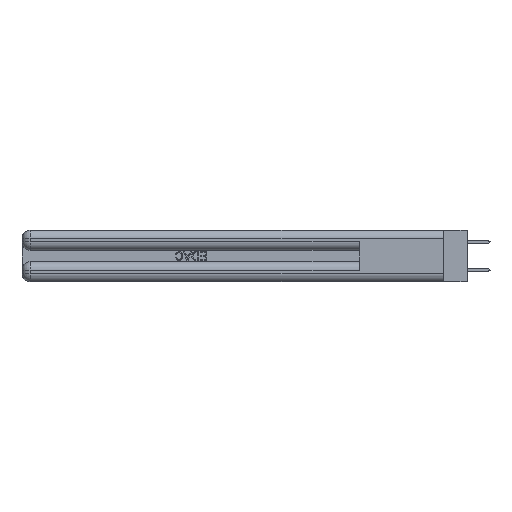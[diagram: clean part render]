
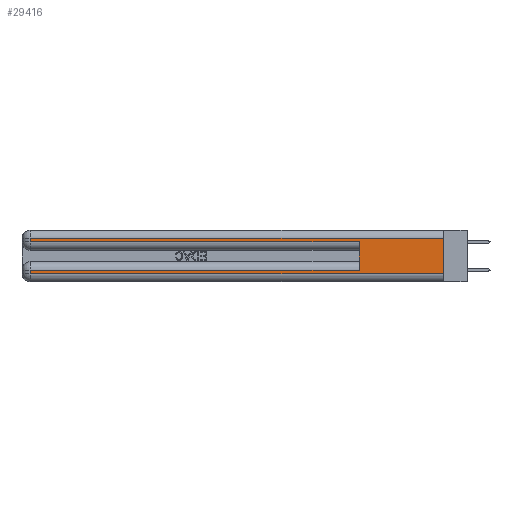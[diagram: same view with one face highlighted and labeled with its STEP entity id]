
A CAD part, left-side view. The second image highlights one B-rep face of the part: STEP entity #29416.
In plain terms, the highlighted planar face has unit normal (-1, 0, 0).
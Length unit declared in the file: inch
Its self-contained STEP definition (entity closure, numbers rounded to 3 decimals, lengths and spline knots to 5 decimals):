
#1865 = EDGE_CURVE ( 'NONE', #43558, #9555, #14047, .T. ) ;
#2271 = AXIS2_PLACEMENT_3D ( 'NONE', #34274, #13079, #16820 ) ;
#2490 = VERTEX_POINT ( 'NONE', #23198 ) ;
#3657 = DIRECTION ( 'NONE',  ( 0., -1., 0. ) ) ;
#5182 = VECTOR ( 'NONE', #38773, 39.37008 ) ;
#5580 = CARTESIAN_POINT ( 'NONE',  ( 0., 0., 0.31 ) ) ;
#7003 = LINE ( 'NONE', #28670, #10877 ) ;
#7326 = ORIENTED_EDGE ( 'NONE', *, *, #19585, .T. ) ;
#7489 = LINE ( 'NONE', #20297, #21971 ) ;
#7851 = DIRECTION ( 'NONE',  ( 0., 0., -1. ) ) ;
#9555 = VERTEX_POINT ( 'NONE', #19583 ) ;
#9772 = VECTOR ( 'NONE', #13461, 39.37008 ) ;
#10008 = CARTESIAN_POINT ( 'NONE',  ( 0., 0.6, 0.085 ) ) ;
#10312 = EDGE_CURVE ( 'NONE', #43558, #22342, #7489, .T. ) ;
#10806 = LINE ( 'NONE', #34805, #19724 ) ;
#10877 = VECTOR ( 'NONE', #35688, 39.37008 ) ;
#13079 = DIRECTION ( 'NONE',  ( 1., 0., 0. ) ) ;
#13461 = DIRECTION ( 'NONE',  ( 0., 0., -1. ) ) ;
#14047 = LINE ( 'NONE', #35183, #5182 ) ;
#14263 = VERTEX_POINT ( 'NONE', #40095 ) ;
#14584 = VERTEX_POINT ( 'NONE', #35047 ) ;
#15767 = CARTESIAN_POINT ( 'NONE',  ( 0., 0., 0.285 ) ) ;
#16317 = EDGE_CURVE ( 'NONE', #22370, #2490, #40449, .T. ) ;
#16820 = DIRECTION ( 'NONE',  ( 0., 0., -1. ) ) ;
#18293 = EDGE_LOOP ( 'NONE', ( #20449, #34323, #7326, #18377, #27210, #22545, #32765, #32266 ) ) ;
#18377 = ORIENTED_EDGE ( 'NONE', *, *, #45230, .T. ) ;
#19583 = CARTESIAN_POINT ( 'NONE',  ( 0., 2.94, 0.085 ) ) ;
#19585 = EDGE_CURVE ( 'NONE', #14263, #36595, #7003, .T. ) ;
#19724 = VECTOR ( 'NONE', #21113, 39.37008 ) ;
#19746 = CARTESIAN_POINT ( 'NONE',  ( 0., 0.6, 0.285 ) ) ;
#20297 = CARTESIAN_POINT ( 'NONE',  ( 0., 0.6, 0.145 ) ) ;
#20449 = ORIENTED_EDGE ( 'NONE', *, *, #16317, .F. ) ;
#20523 = FACE_OUTER_BOUND ( 'NONE', #18293, .T. ) ;
#20891 = DIRECTION ( 'NONE',  ( 0., 0., 1. ) ) ;
#21113 = DIRECTION ( 'NONE',  ( 0., 1., 0. ) ) ;
#21935 = EDGE_CURVE ( 'NONE', #14584, #2490, #26916, .T. ) ;
#21971 = VECTOR ( 'NONE', #20891, 39.37008 ) ;
#22342 = VERTEX_POINT ( 'NONE', #19746 ) ;
#22370 = VERTEX_POINT ( 'NONE', #5580 ) ;
#22545 = ORIENTED_EDGE ( 'NONE', *, *, #1865, .T. ) ;
#23198 = CARTESIAN_POINT ( 'NONE',  ( 0., 0., 0.06 ) ) ;
#24829 = LINE ( 'NONE', #39782, #37623 ) ;
#26690 = DIRECTION ( 'NONE',  ( 0., -1., 0. ) ) ;
#26916 = LINE ( 'NONE', #28413, #43666 ) ;
#27210 = ORIENTED_EDGE ( 'NONE', *, *, #10312, .F. ) ;
#28041 = VECTOR ( 'NONE', #26690, 39.37008 ) ;
#28413 = CARTESIAN_POINT ( 'NONE',  ( 0., 0., 0.06 ) ) ;
#28670 = CARTESIAN_POINT ( 'NONE',  ( 0., 2.94, 0.37 ) ) ;
#29416 = ADVANCED_FACE ( 'NONE', ( #20523 ), #31133, .F. ) ;
#30878 = EDGE_CURVE ( 'NONE', #9555, #14584, #24829, .T. ) ;
#31133 = PLANE ( 'NONE',  #2271 ) ;
#31580 = EDGE_CURVE ( 'NONE', #22370, #14263, #10806, .T. ) ;
#32266 = ORIENTED_EDGE ( 'NONE', *, *, #21935, .T. ) ;
#32765 = ORIENTED_EDGE ( 'NONE', *, *, #30878, .T. ) ;
#34274 = CARTESIAN_POINT ( 'NONE',  ( 0., 0., 0.37 ) ) ;
#34323 = ORIENTED_EDGE ( 'NONE', *, *, #31580, .T. ) ;
#34805 = CARTESIAN_POINT ( 'NONE',  ( 0., 0., 0.31 ) ) ;
#35047 = CARTESIAN_POINT ( 'NONE',  ( 0., 2.94, 0.06 ) ) ;
#35183 = CARTESIAN_POINT ( 'NONE',  ( 0., 0., 0.085 ) ) ;
#35688 = DIRECTION ( 'NONE',  ( 0., 0., -1. ) ) ;
#36595 = VERTEX_POINT ( 'NONE', #39949 ) ;
#37623 = VECTOR ( 'NONE', #7851, 39.37008 ) ;
#38773 = DIRECTION ( 'NONE',  ( 0., 1., 0. ) ) ;
#39782 = CARTESIAN_POINT ( 'NONE',  ( 0., 2.94, 0.37 ) ) ;
#39949 = CARTESIAN_POINT ( 'NONE',  ( 0., 2.94, 0.285 ) ) ;
#40095 = CARTESIAN_POINT ( 'NONE',  ( 0., 2.94, 0.31 ) ) ;
#40449 = LINE ( 'NONE', #45594, #9772 ) ;
#43558 = VERTEX_POINT ( 'NONE', #10008 ) ;
#43666 = VECTOR ( 'NONE', #3657, 39.37008 ) ;
#43712 = LINE ( 'NONE', #15767, #28041 ) ;
#45230 = EDGE_CURVE ( 'NONE', #36595, #22342, #43712, .T. ) ;
#45594 = CARTESIAN_POINT ( 'NONE',  ( 0., 0., 0.37 ) ) ;
